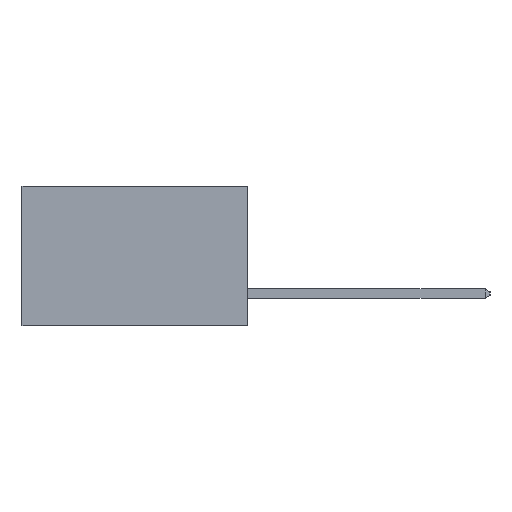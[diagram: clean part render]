
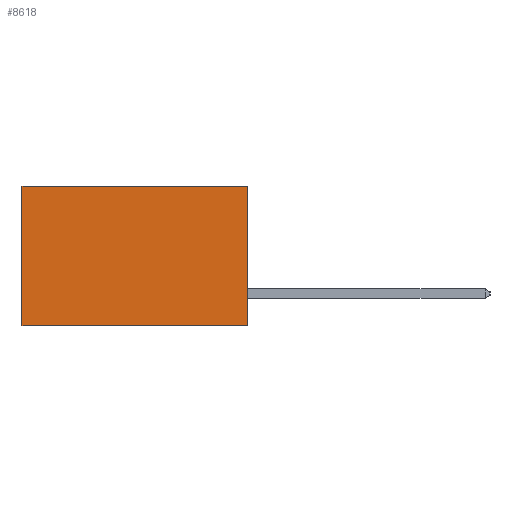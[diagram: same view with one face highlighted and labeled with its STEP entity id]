
A CAD part, left-side view. The second image highlights one B-rep face of the part: STEP entity #8618.
In plain terms, the highlighted planar face has unit normal (-1, 0, 0).
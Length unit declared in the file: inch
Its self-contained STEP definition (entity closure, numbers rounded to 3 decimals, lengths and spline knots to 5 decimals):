
#556 = VERTEX_POINT ( 'NONE', #14922 ) ;
#566 = ORIENTED_EDGE ( 'NONE', *, *, #15171, .T. ) ;
#886 = ORIENTED_EDGE ( 'NONE', *, *, #10796, .T. ) ;
#1964 = CARTESIAN_POINT ( 'NONE',  ( 0.298, 0., -0.37 ) ) ;
#1996 = CARTESIAN_POINT ( 'NONE',  ( 0.298, 0., 0. ) ) ;
#2742 = DIRECTION ( 'NONE',  ( 1., 0., 0. ) ) ;
#2792 = DIRECTION ( 'NONE',  ( 0., 1., 0. ) ) ;
#2869 = VERTEX_POINT ( 'NONE', #1996 ) ;
#4543 = LINE ( 'NONE', #1964, #9600 ) ;
#5190 = CARTESIAN_POINT ( 'NONE',  ( 0.298, 0., 0. ) ) ;
#5987 = CARTESIAN_POINT ( 'NONE',  ( 0.298, 0.6, -0.37 ) ) ;
#6157 = LINE ( 'NONE', #17204, #13804 ) ;
#6615 = VERTEX_POINT ( 'NONE', #5987 ) ;
#6904 = ORIENTED_EDGE ( 'NONE', *, *, #8231, .F. ) ;
#8231 = EDGE_CURVE ( 'NONE', #11634, #6615, #4543, .T. ) ;
#8588 = LINE ( 'NONE', #19656, #12654 ) ;
#8618 = ADVANCED_FACE ( 'NONE', ( #9086 ), #13399, .F. ) ;
#8776 = ORIENTED_EDGE ( 'NONE', *, *, #13042, .F. ) ;
#9086 = FACE_OUTER_BOUND ( 'NONE', #15099, .T. ) ;
#9600 = VECTOR ( 'NONE', #12702, 39.37008 ) ;
#10796 = EDGE_CURVE ( 'NONE', #556, #6615, #6157, .T. ) ;
#11634 = VERTEX_POINT ( 'NONE', #12540 ) ;
#11942 = CARTESIAN_POINT ( 'NONE',  ( 0.298, 0., 0. ) ) ;
#12540 = CARTESIAN_POINT ( 'NONE',  ( 0.298, 0., -0.37 ) ) ;
#12654 = VECTOR ( 'NONE', #2792, 39.37008 ) ;
#12702 = DIRECTION ( 'NONE',  ( 0., 1., 0. ) ) ;
#13042 = EDGE_CURVE ( 'NONE', #2869, #11634, #18805, .T. ) ;
#13399 = PLANE ( 'NONE',  #19653 ) ;
#13462 = DIRECTION ( 'NONE',  ( 0., 0., -1. ) ) ;
#13804 = VECTOR ( 'NONE', #18778, 39.37008 ) ;
#14215 = VECTOR ( 'NONE', #15869, 39.37008 ) ;
#14922 = CARTESIAN_POINT ( 'NONE',  ( 0.298, 0.6, 0. ) ) ;
#15099 = EDGE_LOOP ( 'NONE', ( #886, #6904, #8776, #566 ) ) ;
#15171 = EDGE_CURVE ( 'NONE', #2869, #556, #8588, .T. ) ;
#15869 = DIRECTION ( 'NONE',  ( 0., 0., -1. ) ) ;
#17204 = CARTESIAN_POINT ( 'NONE',  ( 0.298, 0.6, 0. ) ) ;
#18778 = DIRECTION ( 'NONE',  ( 0., 0., -1. ) ) ;
#18805 = LINE ( 'NONE', #5190, #14215 ) ;
#19653 = AXIS2_PLACEMENT_3D ( 'NONE', #11942, #2742, #13462 ) ;
#19656 = CARTESIAN_POINT ( 'NONE',  ( 0.298, 0., 0. ) ) ;
